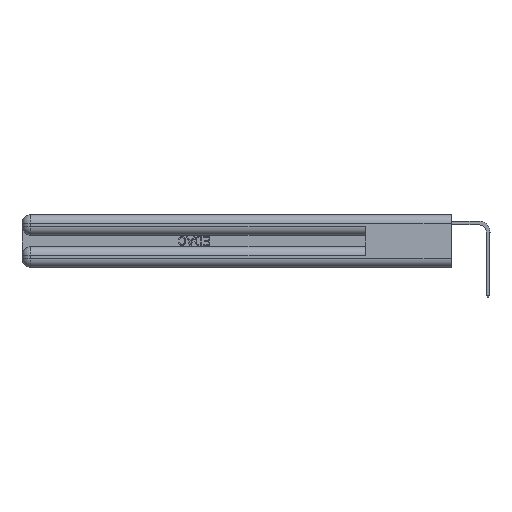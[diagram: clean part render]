
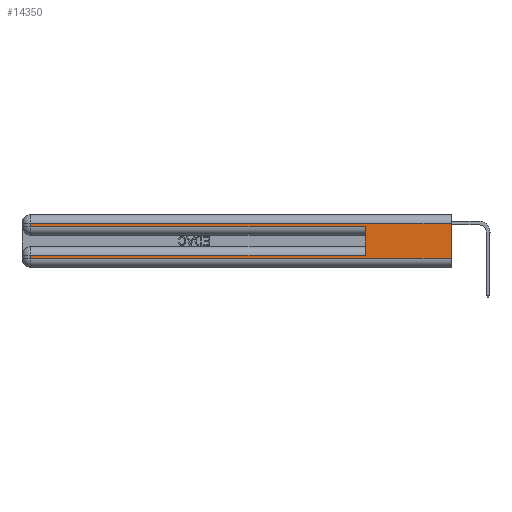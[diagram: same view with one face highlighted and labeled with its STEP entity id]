
A CAD part, left-side view. The second image highlights one B-rep face of the part: STEP entity #14350.
In plain terms, the highlighted planar face has unit normal (-1, 0, 0).
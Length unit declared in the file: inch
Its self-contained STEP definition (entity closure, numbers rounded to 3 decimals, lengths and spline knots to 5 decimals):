
#30 = CARTESIAN_POINT ( 'NONE',  ( 0., 2.94, 0.285 ) ) ;
#458 = DIRECTION ( 'NONE',  ( 0., -1., 0. ) ) ;
#1528 = PLANE ( 'NONE',  #7784 ) ;
#2824 = VECTOR ( 'NONE', #15893, 39.37008 ) ;
#4027 = VECTOR ( 'NONE', #11959, 39.37008 ) ;
#4192 = VERTEX_POINT ( 'NONE', #28413 ) ;
#4815 = CARTESIAN_POINT ( 'NONE',  ( 0., 0.6, 0.285 ) ) ;
#4891 = LINE ( 'NONE', #22105, #4027 ) ;
#5110 = ORIENTED_EDGE ( 'NONE', *, *, #31243, .T. ) ;
#6190 = EDGE_CURVE ( 'NONE', #7503, #24227, #26168, .T. ) ;
#6467 = CARTESIAN_POINT ( 'NONE',  ( 0., 0., 0.31 ) ) ;
#7144 = CARTESIAN_POINT ( 'NONE',  ( 0., 0., 0.085 ) ) ;
#7503 = VERTEX_POINT ( 'NONE', #15623 ) ;
#7621 = ORIENTED_EDGE ( 'NONE', *, *, #28985, .T. ) ;
#7625 = ORIENTED_EDGE ( 'NONE', *, *, #20550, .F. ) ;
#7784 = AXIS2_PLACEMENT_3D ( 'NONE', #31049, #15106, #33730 ) ;
#9129 = EDGE_CURVE ( 'NONE', #28558, #10191, #16105, .T. ) ;
#9805 = EDGE_CURVE ( 'NONE', #15995, #7503, #22711, .T. ) ;
#9975 = VECTOR ( 'NONE', #27816, 39.37008 ) ;
#10191 = VERTEX_POINT ( 'NONE', #20184 ) ;
#10818 = DIRECTION ( 'NONE',  ( 0., 0., -1. ) ) ;
#11959 = DIRECTION ( 'NONE',  ( 0., 0., -1. ) ) ;
#12849 = CARTESIAN_POINT ( 'NONE',  ( 0., 2.94, 0.06 ) ) ;
#14350 = ADVANCED_FACE ( 'NONE', ( #29908 ), #1528, .F. ) ;
#15106 = DIRECTION ( 'NONE',  ( 1., 0., 0. ) ) ;
#15623 = CARTESIAN_POINT ( 'NONE',  ( 0., 2.94, 0.085 ) ) ;
#15893 = DIRECTION ( 'NONE',  ( 0., -1., 0. ) ) ;
#15995 = VERTEX_POINT ( 'NONE', #24270 ) ;
#16105 = LINE ( 'NONE', #6467, #28572 ) ;
#16619 = CARTESIAN_POINT ( 'NONE',  ( 0., 0., 0.06 ) ) ;
#16814 = LINE ( 'NONE', #22959, #30115 ) ;
#17156 = LINE ( 'NONE', #16619, #18846 ) ;
#18115 = EDGE_CURVE ( 'NONE', #28558, #4192, #16814, .T. ) ;
#18846 = VECTOR ( 'NONE', #458, 39.37008 ) ;
#18874 = VERTEX_POINT ( 'NONE', #4815 ) ;
#19360 = ORIENTED_EDGE ( 'NONE', *, *, #6190, .T. ) ;
#20184 = CARTESIAN_POINT ( 'NONE',  ( 0., 2.94, 0.31 ) ) ;
#20550 = EDGE_CURVE ( 'NONE', #15995, #18874, #24173, .T. ) ;
#20569 = ORIENTED_EDGE ( 'NONE', *, *, #9805, .T. ) ;
#21002 = ORIENTED_EDGE ( 'NONE', *, *, #29445, .T. ) ;
#21583 = EDGE_LOOP ( 'NONE', ( #29693, #25987, #5110, #21002, #7625, #20569, #19360, #7621 ) ) ;
#22105 = CARTESIAN_POINT ( 'NONE',  ( 0., 2.94, 0.37 ) ) ;
#22494 = DIRECTION ( 'NONE',  ( 0., 1., 0. ) ) ;
#22711 = LINE ( 'NONE', #7144, #28925 ) ;
#22935 = CARTESIAN_POINT ( 'NONE',  ( 0., 0., 0.31 ) ) ;
#22959 = CARTESIAN_POINT ( 'NONE',  ( 0., 0., 0.37 ) ) ;
#23906 = VERTEX_POINT ( 'NONE', #30 ) ;
#24173 = LINE ( 'NONE', #25172, #9975 ) ;
#24208 = LINE ( 'NONE', #29136, #2824 ) ;
#24227 = VERTEX_POINT ( 'NONE', #12849 ) ;
#24270 = CARTESIAN_POINT ( 'NONE',  ( 0., 0.6, 0.085 ) ) ;
#25172 = CARTESIAN_POINT ( 'NONE',  ( 0., 0.6, 0.145 ) ) ;
#25634 = DIRECTION ( 'NONE',  ( 0., 0., -1. ) ) ;
#25987 = ORIENTED_EDGE ( 'NONE', *, *, #9129, .T. ) ;
#26168 = LINE ( 'NONE', #32135, #32407 ) ;
#27816 = DIRECTION ( 'NONE',  ( 0., 0., 1. ) ) ;
#28413 = CARTESIAN_POINT ( 'NONE',  ( 0., 0., 0.06 ) ) ;
#28558 = VERTEX_POINT ( 'NONE', #22935 ) ;
#28572 = VECTOR ( 'NONE', #22494, 39.37008 ) ;
#28925 = VECTOR ( 'NONE', #33862, 39.37008 ) ;
#28985 = EDGE_CURVE ( 'NONE', #24227, #4192, #17156, .T. ) ;
#29136 = CARTESIAN_POINT ( 'NONE',  ( 0., 0., 0.285 ) ) ;
#29445 = EDGE_CURVE ( 'NONE', #23906, #18874, #24208, .T. ) ;
#29693 = ORIENTED_EDGE ( 'NONE', *, *, #18115, .F. ) ;
#29908 = FACE_OUTER_BOUND ( 'NONE', #21583, .T. ) ;
#30115 = VECTOR ( 'NONE', #25634, 39.37008 ) ;
#31049 = CARTESIAN_POINT ( 'NONE',  ( 0., 0., 0.37 ) ) ;
#31243 = EDGE_CURVE ( 'NONE', #10191, #23906, #4891, .T. ) ;
#32135 = CARTESIAN_POINT ( 'NONE',  ( 0., 2.94, 0.37 ) ) ;
#32407 = VECTOR ( 'NONE', #10818, 39.37008 ) ;
#33730 = DIRECTION ( 'NONE',  ( 0., 0., -1. ) ) ;
#33862 = DIRECTION ( 'NONE',  ( 0., 1., 0. ) ) ;
